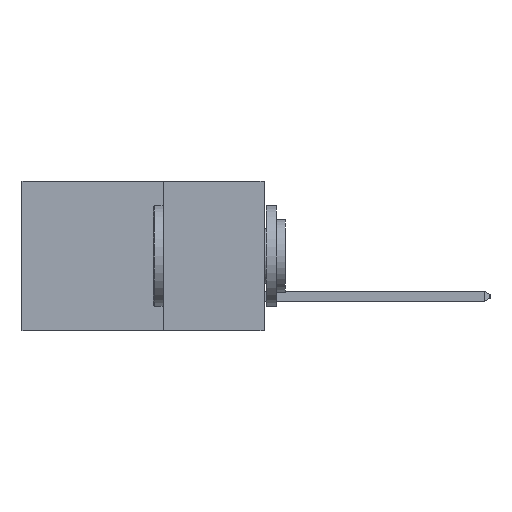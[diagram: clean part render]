
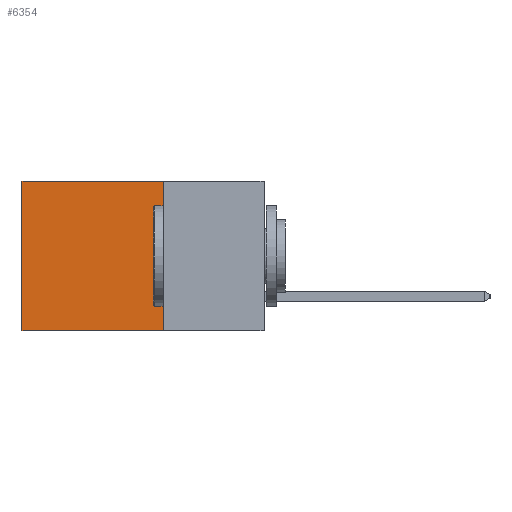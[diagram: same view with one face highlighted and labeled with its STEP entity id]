
A CAD part, left-side view. The second image highlights one B-rep face of the part: STEP entity #6354.
In plain terms, the highlighted planar face has unit normal (-1, 0, 0).
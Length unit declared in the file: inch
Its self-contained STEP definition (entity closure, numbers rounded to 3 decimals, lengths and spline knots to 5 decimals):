
#9 = LINE ( 'NONE', #11669, #3218 ) ;
#12 = EDGE_CURVE ( 'NONE', #347, #1405, #4068, .T. ) ;
#82 = EDGE_CURVE ( 'NONE', #1525, #347, #4200, .T. ) ;
#347 = VERTEX_POINT ( 'NONE', #5374 ) ;
#1279 = DIRECTION ( 'NONE',  ( 0., 1., 0. ) ) ;
#1405 = VERTEX_POINT ( 'NONE', #3723 ) ;
#1463 = VECTOR ( 'NONE', #1279, 39.37008 ) ;
#1525 = VERTEX_POINT ( 'NONE', #11727 ) ;
#1760 = DIRECTION ( 'NONE',  ( 0., 1., 0. ) ) ;
#2066 = ORIENTED_EDGE ( 'NONE', *, *, #12, .T. ) ;
#2069 = ORIENTED_EDGE ( 'NONE', *, *, #7845, .F. ) ;
#2082 = ORIENTED_EDGE ( 'NONE', *, *, #2716, .F. ) ;
#2086 = ORIENTED_EDGE ( 'NONE', *, *, #82, .T. ) ;
#2318 = VECTOR ( 'NONE', #1760, 39.37008 ) ;
#2716 = EDGE_CURVE ( 'NONE', #1525, #2835, #9, .T. ) ;
#2835 = VERTEX_POINT ( 'NONE', #9736 ) ;
#3218 = VECTOR ( 'NONE', #11655, 39.37008 ) ;
#3723 = CARTESIAN_POINT ( 'NONE',  ( 0.2615, 0.6, -0.37 ) ) ;
#3941 = DIRECTION ( 'NONE',  ( 0., 0., -1. ) ) ;
#4068 = LINE ( 'NONE', #10144, #8586 ) ;
#4200 = LINE ( 'NONE', #8332, #1463 ) ;
#4531 = CARTESIAN_POINT ( 'NONE',  ( 0.2615, 0.25, -0.37 ) ) ;
#4966 = LINE ( 'NONE', #9543, #2318 ) ;
#5374 = CARTESIAN_POINT ( 'NONE',  ( 0.2615, 0.6, 0. ) ) ;
#5478 = DIRECTION ( 'NONE',  ( 0., 0., -1. ) ) ;
#5838 = EDGE_LOOP ( 'NONE', ( #2066, #2069, #2082, #2086 ) ) ;
#6354 = ADVANCED_FACE ( 'NONE', ( #6377 ), #10126, .F. ) ;
#6377 = FACE_OUTER_BOUND ( 'NONE', #5838, .T. ) ;
#7845 = EDGE_CURVE ( 'NONE', #2835, #1405, #4966, .T. ) ;
#8332 = CARTESIAN_POINT ( 'NONE',  ( 0.2615, 0.25, 0. ) ) ;
#8586 = VECTOR ( 'NONE', #3941, 39.37008 ) ;
#9543 = CARTESIAN_POINT ( 'NONE',  ( 0.2615, 0.25, -0.37 ) ) ;
#9736 = CARTESIAN_POINT ( 'NONE',  ( 0.2615, 0.25, -0.37 ) ) ;
#10126 = PLANE ( 'NONE',  #11882 ) ;
#10144 = CARTESIAN_POINT ( 'NONE',  ( 0.2615, 0.6, -0.37 ) ) ;
#10956 = DIRECTION ( 'NONE',  ( 1., 0., 0. ) ) ;
#11655 = DIRECTION ( 'NONE',  ( 0., 0., -1. ) ) ;
#11669 = CARTESIAN_POINT ( 'NONE',  ( 0.2615, 0.25, -0.37 ) ) ;
#11727 = CARTESIAN_POINT ( 'NONE',  ( 0.2615, 0.25, 0. ) ) ;
#11882 = AXIS2_PLACEMENT_3D ( 'NONE', #4531, #10956, #5478 ) ;
